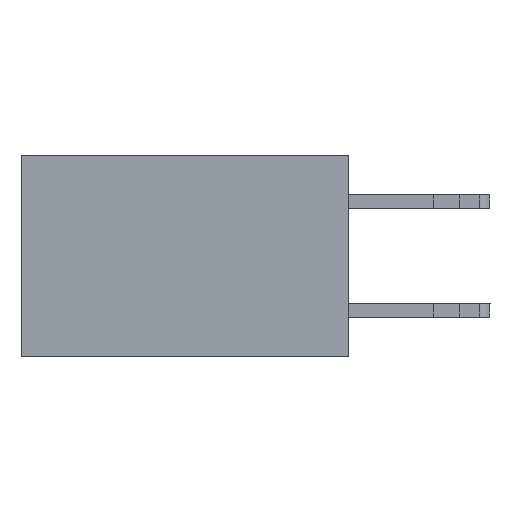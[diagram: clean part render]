
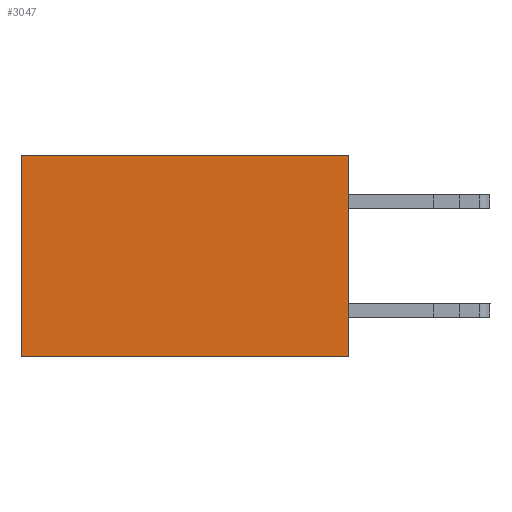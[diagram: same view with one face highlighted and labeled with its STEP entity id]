
A CAD part, left-side view. The second image highlights one B-rep face of the part: STEP entity #3047.
In plain terms, the highlighted planar face has unit normal (-1, 0, 0).
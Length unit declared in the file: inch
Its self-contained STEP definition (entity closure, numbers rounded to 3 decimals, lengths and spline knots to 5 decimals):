
#108 = VECTOR ( 'NONE', #6667, 39.37008 ) ;
#237 = VERTEX_POINT ( 'NONE', #7467 ) ;
#734 = CARTESIAN_POINT ( 'NONE',  ( 0.2615, 0., -0.37 ) ) ;
#887 = VERTEX_POINT ( 'NONE', #11259 ) ;
#1727 = EDGE_CURVE ( 'NONE', #887, #10385, #8242, .T. ) ;
#1778 = VECTOR ( 'NONE', #5672, 39.37008 ) ;
#2172 = LINE ( 'NONE', #6049, #12381 ) ;
#2588 = EDGE_CURVE ( 'NONE', #887, #237, #2172, .T. ) ;
#2964 = EDGE_CURVE ( 'NONE', #237, #11172, #8118, .T. ) ;
#3047 = ADVANCED_FACE ( 'NONE', ( #4143 ), #3287, .F. ) ;
#3287 = PLANE ( 'NONE',  #10124 ) ;
#3460 = DIRECTION ( 'NONE',  ( 1., 0., 0. ) ) ;
#3614 = DIRECTION ( 'NONE',  ( 0., 0., -1. ) ) ;
#3689 = CARTESIAN_POINT ( 'NONE',  ( 0.2615, 0., -0.37 ) ) ;
#3949 = DIRECTION ( 'NONE',  ( 0., 0., -1. ) ) ;
#4143 = FACE_OUTER_BOUND ( 'NONE', #5147, .T. ) ;
#4182 = CARTESIAN_POINT ( 'NONE',  ( 0.2615, 0., -0.37 ) ) ;
#4685 = LINE ( 'NONE', #734, #1778 ) ;
#4968 = ORIENTED_EDGE ( 'NONE', *, *, #10687, .F. ) ;
#5147 = EDGE_LOOP ( 'NONE', ( #8507, #4968, #5953, #9841 ) ) ;
#5672 = DIRECTION ( 'NONE',  ( 0., 1., 0. ) ) ;
#5766 = CARTESIAN_POINT ( 'NONE',  ( 0.2615, 0., -0.37 ) ) ;
#5953 = ORIENTED_EDGE ( 'NONE', *, *, #1727, .F. ) ;
#6049 = CARTESIAN_POINT ( 'NONE',  ( 0.2615, 0., 0. ) ) ;
#6667 = DIRECTION ( 'NONE',  ( 0., 0., -1. ) ) ;
#7467 = CARTESIAN_POINT ( 'NONE',  ( 0.2615, 0.6, 0. ) ) ;
#8118 = LINE ( 'NONE', #8441, #108 ) ;
#8242 = LINE ( 'NONE', #5766, #10294 ) ;
#8441 = CARTESIAN_POINT ( 'NONE',  ( 0.2615, 0.6, -0.37 ) ) ;
#8507 = ORIENTED_EDGE ( 'NONE', *, *, #2964, .T. ) ;
#8556 = CARTESIAN_POINT ( 'NONE',  ( 0.2615, 0.6, -0.37 ) ) ;
#9171 = DIRECTION ( 'NONE',  ( 0., 1., 0. ) ) ;
#9841 = ORIENTED_EDGE ( 'NONE', *, *, #2588, .T. ) ;
#10124 = AXIS2_PLACEMENT_3D ( 'NONE', #3689, #3460, #3949 ) ;
#10294 = VECTOR ( 'NONE', #3614, 39.37008 ) ;
#10385 = VERTEX_POINT ( 'NONE', #4182 ) ;
#10687 = EDGE_CURVE ( 'NONE', #10385, #11172, #4685, .T. ) ;
#11172 = VERTEX_POINT ( 'NONE', #8556 ) ;
#11259 = CARTESIAN_POINT ( 'NONE',  ( 0.2615, 0., 0. ) ) ;
#12381 = VECTOR ( 'NONE', #9171, 39.37008 ) ;
